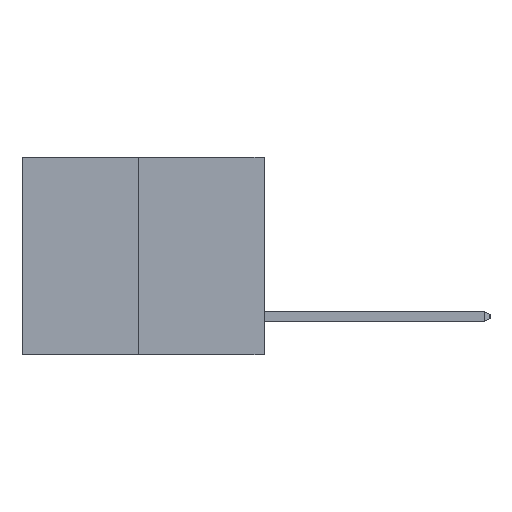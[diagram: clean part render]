
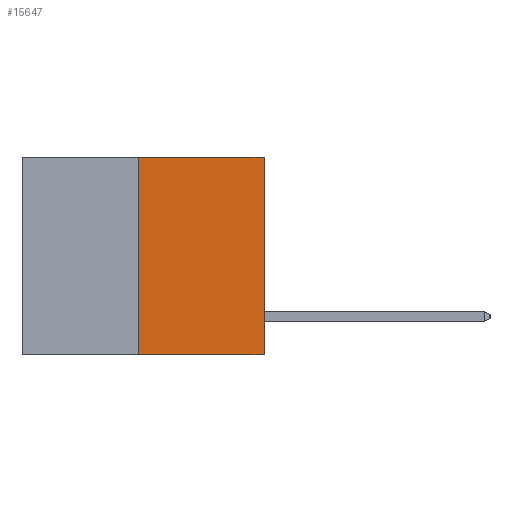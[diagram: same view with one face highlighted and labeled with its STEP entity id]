
A CAD part, left-side view. The second image highlights one B-rep face of the part: STEP entity #15647.
In plain terms, the highlighted planar face has unit normal (-1, 0, 0).
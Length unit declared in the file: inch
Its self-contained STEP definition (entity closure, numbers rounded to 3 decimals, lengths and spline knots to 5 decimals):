
#239 = VERTEX_POINT ( 'NONE', #17001 ) ;
#528 = DIRECTION ( 'NONE',  ( 0., 0., -1. ) ) ;
#1966 = EDGE_LOOP ( 'NONE', ( #15542, #23101, #18547, #8753 ) ) ;
#2394 = CARTESIAN_POINT ( 'NONE',  ( 0., 0.6, 0. ) ) ;
#3556 = DIRECTION ( 'NONE',  ( 0., 0., 1. ) ) ;
#3822 = DIRECTION ( 'NONE',  ( 0., -1., 0. ) ) ;
#4736 = VECTOR ( 'NONE', #3822, 39.37008 ) ;
#5082 = VECTOR ( 'NONE', #20518, 39.37008 ) ;
#5875 = VECTOR ( 'NONE', #24680, 39.37008 ) ;
#6625 = EDGE_CURVE ( 'NONE', #9703, #15884, #14514, .T. ) ;
#7467 = CARTESIAN_POINT ( 'NONE',  ( 0., 0.312, -0.49 ) ) ;
#7515 = LINE ( 'NONE', #16427, #18600 ) ;
#7582 = EDGE_CURVE ( 'NONE', #9782, #239, #13092, .T. ) ;
#8753 = ORIENTED_EDGE ( 'NONE', *, *, #6625, .F. ) ;
#9703 = VERTEX_POINT ( 'NONE', #21826 ) ;
#9782 = VERTEX_POINT ( 'NONE', #26251 ) ;
#10150 = FACE_OUTER_BOUND ( 'NONE', #1966, .T. ) ;
#11039 = DIRECTION ( 'NONE',  ( 1., 0., 0. ) ) ;
#11569 = LINE ( 'NONE', #7467, #5875 ) ;
#13092 = LINE ( 'NONE', #25459, #4736 ) ;
#13346 = EDGE_CURVE ( 'NONE', #9782, #9703, #11569, .T. ) ;
#14514 = LINE ( 'NONE', #24587, #5082 ) ;
#14519 = EDGE_CURVE ( 'NONE', #239, #15884, #7515, .T. ) ;
#15542 = ORIENTED_EDGE ( 'NONE', *, *, #13346, .F. ) ;
#15647 = ADVANCED_FACE ( 'NONE', ( #10150 ), #21765, .F. ) ;
#15884 = VERTEX_POINT ( 'NONE', #22817 ) ;
#16427 = CARTESIAN_POINT ( 'NONE',  ( 0., 0., 0. ) ) ;
#17001 = CARTESIAN_POINT ( 'NONE',  ( 0., 0., -0.49 ) ) ;
#18547 = ORIENTED_EDGE ( 'NONE', *, *, #14519, .T. ) ;
#18600 = VECTOR ( 'NONE', #3556, 39.37008 ) ;
#20518 = DIRECTION ( 'NONE',  ( 0., -1., 0. ) ) ;
#20684 = AXIS2_PLACEMENT_3D ( 'NONE', #2394, #11039, #528 ) ;
#21765 = PLANE ( 'NONE',  #20684 ) ;
#21826 = CARTESIAN_POINT ( 'NONE',  ( 0., 0.312, 0. ) ) ;
#22817 = CARTESIAN_POINT ( 'NONE',  ( 0., 0., 0. ) ) ;
#23101 = ORIENTED_EDGE ( 'NONE', *, *, #7582, .T. ) ;
#24587 = CARTESIAN_POINT ( 'NONE',  ( 0., 0.6, 0. ) ) ;
#24680 = DIRECTION ( 'NONE',  ( 0., 0., 1. ) ) ;
#25459 = CARTESIAN_POINT ( 'NONE',  ( 0., 0.6, -0.49 ) ) ;
#26251 = CARTESIAN_POINT ( 'NONE',  ( 0., 0.312, -0.49 ) ) ;
